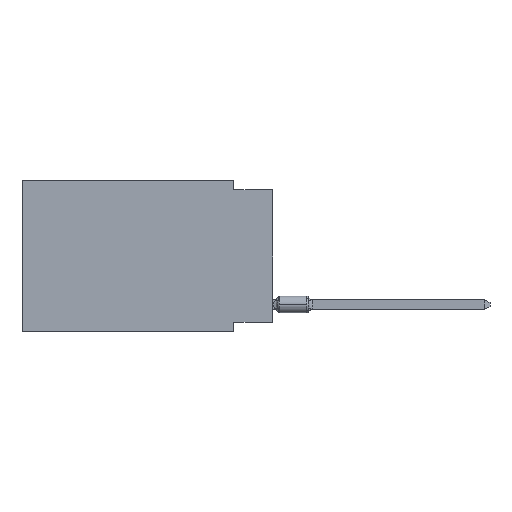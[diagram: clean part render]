
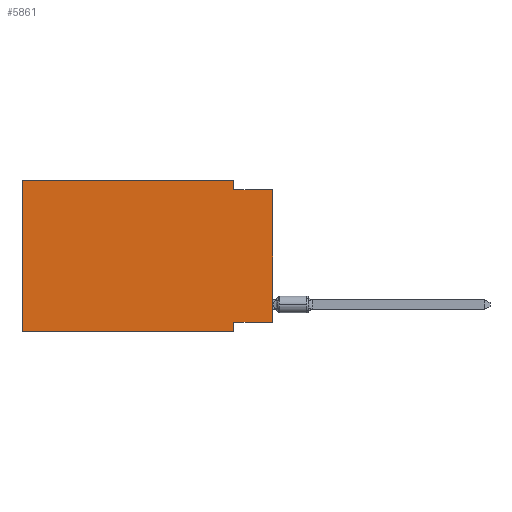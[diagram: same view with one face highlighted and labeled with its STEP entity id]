
A CAD part, left-side view. The second image highlights one B-rep face of the part: STEP entity #5861.
In plain terms, the highlighted planar face has unit normal (-1, 0, 0).
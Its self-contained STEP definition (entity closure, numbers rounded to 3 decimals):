
#129 = LINE ( 'NONE', #7257, #12031 ) ;
#460 = VECTOR ( 'NONE', #4602, 1000. ) ;
#689 = VECTOR ( 'NONE', #7741, 1000. ) ;
#833 = EDGE_CURVE ( 'NONE', #9172, #8712, #4521, .T. ) ;
#834 = DIRECTION ( 'NONE',  ( 0., 0., -1. ) ) ;
#967 = LINE ( 'NONE', #3936, #7565 ) ;
#1072 = EDGE_CURVE ( 'NONE', #5626, #3513, #5395, .T. ) ;
#1203 = FACE_OUTER_BOUND ( 'NONE', #10204, .T. ) ;
#1340 = LINE ( 'NONE', #9242, #6298 ) ;
#1363 = DIRECTION ( 'NONE',  ( 0., 0., -1. ) ) ;
#1542 = CARTESIAN_POINT ( 'NONE',  ( 0., 2.54, 0. ) ) ;
#1558 = EDGE_CURVE ( 'NONE', #9172, #4970, #6679, .T. ) ;
#1610 = VERTEX_POINT ( 'NONE', #8425 ) ;
#1829 = CARTESIAN_POINT ( 'NONE',  ( 0., 0., -9.271 ) ) ;
#2411 = DIRECTION ( 'NONE',  ( 0., 0., 1. ) ) ;
#2451 = LINE ( 'NONE', #1542, #11021 ) ;
#2588 = ORIENTED_EDGE ( 'NONE', *, *, #833, .F. ) ;
#2619 = AXIS2_PLACEMENT_3D ( 'NONE', #5153, #8811, #834 ) ;
#2677 = LINE ( 'NONE', #12438, #689 ) ;
#2778 = ORIENTED_EDGE ( 'NONE', *, *, #5039, .T. ) ;
#3019 = VECTOR ( 'NONE', #2411, 1000. ) ;
#3374 = EDGE_CURVE ( 'NONE', #3513, #12229, #967, .T. ) ;
#3513 = VERTEX_POINT ( 'NONE', #8985 ) ;
#3701 = ORIENTED_EDGE ( 'NONE', *, *, #11908, .F. ) ;
#3861 = VERTEX_POINT ( 'NONE', #7618 ) ;
#3893 = CARTESIAN_POINT ( 'NONE',  ( 0., 16.383, -9.906 ) ) ;
#3936 = CARTESIAN_POINT ( 'NONE',  ( 0., 16.383, 0. ) ) ;
#4311 = DIRECTION ( 'NONE',  ( 0., -1., 0. ) ) ;
#4521 = LINE ( 'NONE', #5422, #11478 ) ;
#4602 = DIRECTION ( 'NONE',  ( 0., 0., 1. ) ) ;
#4754 = ORIENTED_EDGE ( 'NONE', *, *, #1072, .F. ) ;
#4970 = VERTEX_POINT ( 'NONE', #5802 ) ;
#5039 = EDGE_CURVE ( 'NONE', #5626, #1610, #2677, .T. ) ;
#5153 = CARTESIAN_POINT ( 'NONE',  ( 0., 16.383, 0. ) ) ;
#5395 = LINE ( 'NONE', #12038, #3019 ) ;
#5422 = CARTESIAN_POINT ( 'NONE',  ( 0., 0., -9.271 ) ) ;
#5626 = VERTEX_POINT ( 'NONE', #3893 ) ;
#5802 = CARTESIAN_POINT ( 'NONE',  ( 0., 0., -0.635 ) ) ;
#5861 = ADVANCED_FACE ( 'NONE', ( #1203 ), #7101, .F. ) ;
#6281 = ORIENTED_EDGE ( 'NONE', *, *, #1558, .T. ) ;
#6298 = VECTOR ( 'NONE', #4311, 1000. ) ;
#6622 = CARTESIAN_POINT ( 'NONE',  ( 0., 0., 0. ) ) ;
#6679 = LINE ( 'NONE', #6622, #460 ) ;
#6937 = DIRECTION ( 'NONE',  ( 0., -1., 0. ) ) ;
#7101 = PLANE ( 'NONE',  #2619 ) ;
#7257 = CARTESIAN_POINT ( 'NONE',  ( 0., 2.54, -9.906 ) ) ;
#7565 = VECTOR ( 'NONE', #6937, 1000. ) ;
#7618 = CARTESIAN_POINT ( 'NONE',  ( 0., 2.54, -0.635 ) ) ;
#7741 = DIRECTION ( 'NONE',  ( 0., -1., 0. ) ) ;
#8344 = DIRECTION ( 'NONE',  ( 0., 0., -1. ) ) ;
#8425 = CARTESIAN_POINT ( 'NONE',  ( 0., 2.54, -9.906 ) ) ;
#8712 = VERTEX_POINT ( 'NONE', #8800 ) ;
#8780 = ORIENTED_EDGE ( 'NONE', *, *, #11029, .F. ) ;
#8800 = CARTESIAN_POINT ( 'NONE',  ( 0., 2.54, -9.271 ) ) ;
#8811 = DIRECTION ( 'NONE',  ( 1., 0., 0. ) ) ;
#8985 = CARTESIAN_POINT ( 'NONE',  ( 0., 16.383, 0. ) ) ;
#9172 = VERTEX_POINT ( 'NONE', #1829 ) ;
#9242 = CARTESIAN_POINT ( 'NONE',  ( 0., 0., -0.635 ) ) ;
#9375 = DIRECTION ( 'NONE',  ( 0., 1., 0. ) ) ;
#10204 = EDGE_LOOP ( 'NONE', ( #6281, #3701, #8780, #12528, #4754, #2778, #11138, #2588 ) ) ;
#10950 = EDGE_CURVE ( 'NONE', #8712, #1610, #129, .T. ) ;
#11021 = VECTOR ( 'NONE', #8344, 1000. ) ;
#11029 = EDGE_CURVE ( 'NONE', #12229, #3861, #2451, .T. ) ;
#11138 = ORIENTED_EDGE ( 'NONE', *, *, #10950, .F. ) ;
#11384 = CARTESIAN_POINT ( 'NONE',  ( 0., 2.54, 0. ) ) ;
#11478 = VECTOR ( 'NONE', #9375, 1000. ) ;
#11908 = EDGE_CURVE ( 'NONE', #3861, #4970, #1340, .T. ) ;
#12031 = VECTOR ( 'NONE', #1363, 1000. ) ;
#12038 = CARTESIAN_POINT ( 'NONE',  ( 0., 16.383, 0. ) ) ;
#12229 = VERTEX_POINT ( 'NONE', #11384 ) ;
#12438 = CARTESIAN_POINT ( 'NONE',  ( 0., 16.383, -9.906 ) ) ;
#12528 = ORIENTED_EDGE ( 'NONE', *, *, #3374, .F. ) ;
